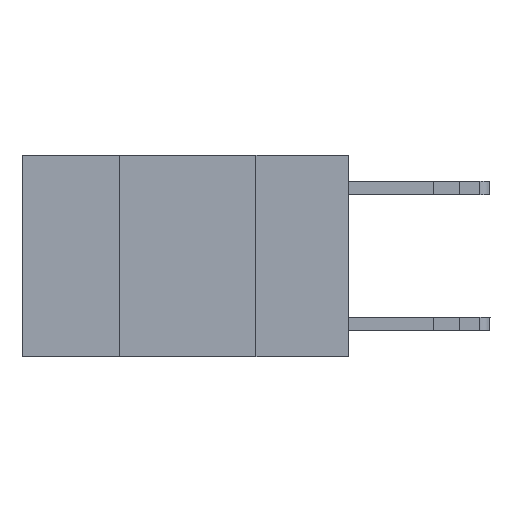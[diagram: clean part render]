
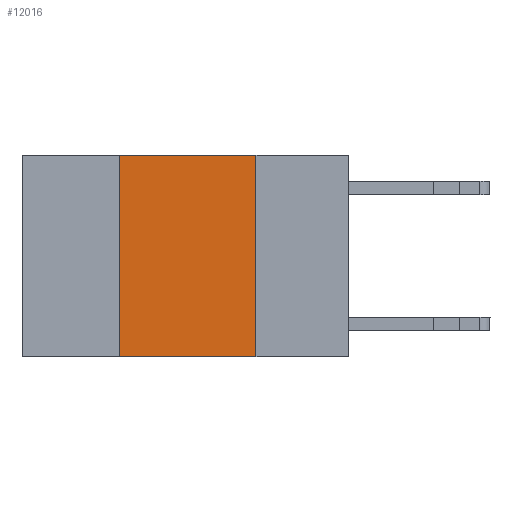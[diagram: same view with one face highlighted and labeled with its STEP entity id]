
A CAD part, left-side view. The second image highlights one B-rep face of the part: STEP entity #12016.
In plain terms, the highlighted planar face has unit normal (-1, 0, 0).
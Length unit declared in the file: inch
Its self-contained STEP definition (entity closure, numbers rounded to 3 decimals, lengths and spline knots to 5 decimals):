
#2115 = VERTEX_POINT ( 'NONE', #3479 ) ;
#2676 = DIRECTION ( 'NONE',  ( 0., 0., -1. ) ) ;
#3179 = CARTESIAN_POINT ( 'NONE',  ( 0., 0.17, 0. ) ) ;
#3323 = DIRECTION ( 'NONE',  ( 0., 0., 1. ) ) ;
#3479 = CARTESIAN_POINT ( 'NONE',  ( 0., 0.17, -0.37 ) ) ;
#3588 = CARTESIAN_POINT ( 'NONE',  ( 0., 0.42, 0. ) ) ;
#3673 = VERTEX_POINT ( 'NONE', #14421 ) ;
#3815 = VECTOR ( 'NONE', #3323, 39.37008 ) ;
#3949 = LINE ( 'NONE', #3588, #3815 ) ;
#4533 = VERTEX_POINT ( 'NONE', #19884 ) ;
#5034 = EDGE_CURVE ( 'NONE', #3673, #2115, #9014, .T. ) ;
#5318 = EDGE_CURVE ( 'NONE', #8519, #4533, #6451, .T. ) ;
#5586 = EDGE_CURVE ( 'NONE', #3673, #8519, #3949, .T. ) ;
#6016 = VECTOR ( 'NONE', #10352, 39.37008 ) ;
#6451 = LINE ( 'NONE', #11192, #6016 ) ;
#8519 = VERTEX_POINT ( 'NONE', #9244 ) ;
#8759 = AXIS2_PLACEMENT_3D ( 'NONE', #16932, #16879, #16767 ) ;
#8858 = VECTOR ( 'NONE', #18372, 39.37008 ) ;
#9014 = LINE ( 'NONE', #18636, #8858 ) ;
#9244 = CARTESIAN_POINT ( 'NONE',  ( 0., 0.42, 0. ) ) ;
#9825 = EDGE_LOOP ( 'NONE', ( #14033, #14586, #14693, #15364 ) ) ;
#10352 = DIRECTION ( 'NONE',  ( 0., -1., 0. ) ) ;
#11192 = CARTESIAN_POINT ( 'NONE',  ( 0., 0.6, 0. ) ) ;
#12016 = ADVANCED_FACE ( 'NONE', ( #14628 ), #16884, .F. ) ;
#14033 = ORIENTED_EDGE ( 'NONE', *, *, #16255, .F. ) ;
#14396 = VECTOR ( 'NONE', #2676, 39.37008 ) ;
#14421 = CARTESIAN_POINT ( 'NONE',  ( 0., 0.42, -0.37 ) ) ;
#14571 = LINE ( 'NONE', #3179, #14396 ) ;
#14586 = ORIENTED_EDGE ( 'NONE', *, *, #5318, .F. ) ;
#14628 = FACE_OUTER_BOUND ( 'NONE', #9825, .T. ) ;
#14693 = ORIENTED_EDGE ( 'NONE', *, *, #5586, .F. ) ;
#15364 = ORIENTED_EDGE ( 'NONE', *, *, #5034, .T. ) ;
#16255 = EDGE_CURVE ( 'NONE', #4533, #2115, #14571, .T. ) ;
#16767 = DIRECTION ( 'NONE',  ( 0., 0., -1. ) ) ;
#16879 = DIRECTION ( 'NONE',  ( 1., 0., 0. ) ) ;
#16884 = PLANE ( 'NONE',  #8759 ) ;
#16932 = CARTESIAN_POINT ( 'NONE',  ( 0., 0.6, 0. ) ) ;
#18372 = DIRECTION ( 'NONE',  ( 0., -1., 0. ) ) ;
#18636 = CARTESIAN_POINT ( 'NONE',  ( 0., 0.6, -0.37 ) ) ;
#19884 = CARTESIAN_POINT ( 'NONE',  ( 0., 0.17, 0. ) ) ;
